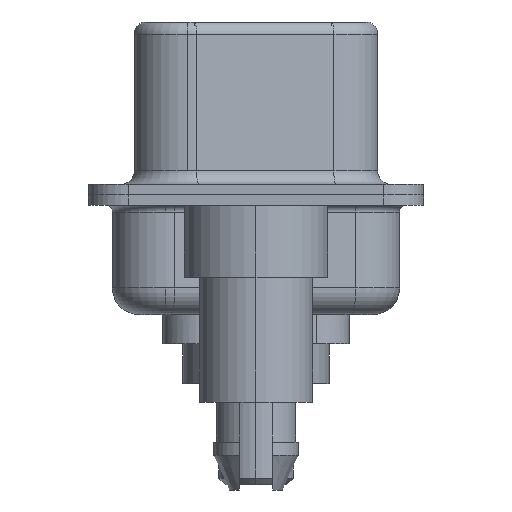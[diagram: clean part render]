
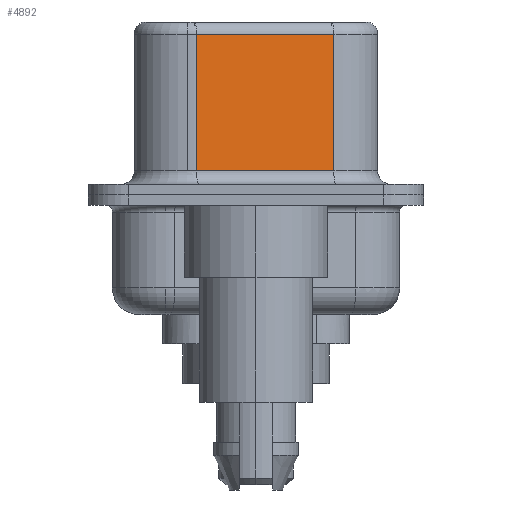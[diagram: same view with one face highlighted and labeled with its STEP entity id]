
A CAD part, left-side view. The second image highlights one B-rep face of the part: STEP entity #4892.
In plain terms, the highlighted planar face has unit normal (-0.985, -0.174, 0).
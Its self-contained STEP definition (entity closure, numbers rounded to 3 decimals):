
#714 = AXIS2_PLACEMENT_3D ( 'NONE', #2386, #7748, #7531 ) ;
#1289 = LINE ( 'NONE', #4062, #3058 ) ;
#1626 = ORIENTED_EDGE ( 'NONE', *, *, #18757, .T. ) ;
#2142 = DIRECTION ( 'NONE',  ( 0., 0., -1. ) ) ;
#2386 = CARTESIAN_POINT ( 'NONE',  ( 4.58, -2.927, 6.52 ) ) ;
#2649 = VERTEX_POINT ( 'NONE', #14355 ) ;
#3058 = VECTOR ( 'NONE', #3908, 1000. ) ;
#3774 = DIRECTION ( 'NONE',  ( 0., 0., -1. ) ) ;
#3908 = DIRECTION ( 'NONE',  ( 0.174, -0.985, 0. ) ) ;
#4062 = CARTESIAN_POINT ( 'NONE',  ( 4.58, -2.927, 0.9 ) ) ;
#4108 = VERTEX_POINT ( 'NONE', #8655 ) ;
#4892 = ADVANCED_FACE ( 'NONE', ( #17048 ), #17200, .F. ) ;
#4964 = CARTESIAN_POINT ( 'NONE',  ( 4.58, -2.927, 0.9 ) ) ;
#5136 = VECTOR ( 'NONE', #16089, 1000. ) ;
#6064 = ORIENTED_EDGE ( 'NONE', *, *, #19702, .T. ) ;
#6077 = VECTOR ( 'NONE', #3774, 1000. ) ;
#7440 = ORIENTED_EDGE ( 'NONE', *, *, #15844, .F. ) ;
#7531 = DIRECTION ( 'NONE',  ( -0.174, 0.985, 0. ) ) ;
#7748 = DIRECTION ( 'NONE',  ( 0.985, 0.174, 0. ) ) ;
#8655 = CARTESIAN_POINT ( 'NONE',  ( 3.67, 2.233, 0.9 ) ) ;
#8785 = LINE ( 'NONE', #19220, #6077 ) ;
#10034 = VERTEX_POINT ( 'NONE', #13989 ) ;
#10981 = EDGE_LOOP ( 'NONE', ( #7440, #1626, #16696, #6064 ) ) ;
#11712 = EDGE_CURVE ( 'NONE', #10034, #4108, #18363, .T. ) ;
#12231 = LINE ( 'NONE', #20851, #5136 ) ;
#13257 = VECTOR ( 'NONE', #2142, 1000. ) ;
#13989 = CARTESIAN_POINT ( 'NONE',  ( 3.67, 2.233, 6.02 ) ) ;
#14355 = CARTESIAN_POINT ( 'NONE',  ( 4.58, -2.927, 6.02 ) ) ;
#15361 = CARTESIAN_POINT ( 'NONE',  ( 3.67, 2.233, 6.52 ) ) ;
#15844 = EDGE_CURVE ( 'NONE', #2649, #15925, #8785, .T. ) ;
#15925 = VERTEX_POINT ( 'NONE', #4964 ) ;
#16089 = DIRECTION ( 'NONE',  ( -0.174, 0.985, 0. ) ) ;
#16696 = ORIENTED_EDGE ( 'NONE', *, *, #11712, .T. ) ;
#17048 = FACE_OUTER_BOUND ( 'NONE', #10981, .T. ) ;
#17200 = PLANE ( 'NONE',  #714 ) ;
#18363 = LINE ( 'NONE', #15361, #13257 ) ;
#18757 = EDGE_CURVE ( 'NONE', #2649, #10034, #12231, .T. ) ;
#19220 = CARTESIAN_POINT ( 'NONE',  ( 4.58, -2.927, 6.52 ) ) ;
#19702 = EDGE_CURVE ( 'NONE', #4108, #15925, #1289, .T. ) ;
#20851 = CARTESIAN_POINT ( 'NONE',  ( 4.58, -2.927, 6.02 ) ) ;
